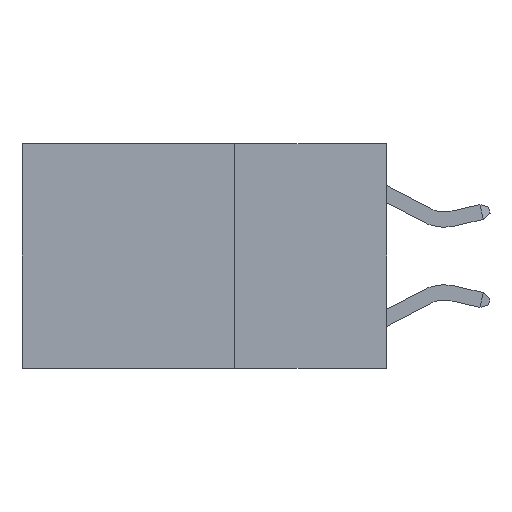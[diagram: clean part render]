
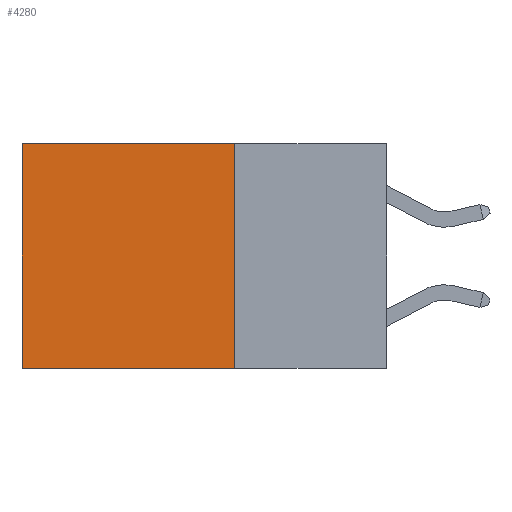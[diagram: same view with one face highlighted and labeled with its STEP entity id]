
A CAD part, left-side view. The second image highlights one B-rep face of the part: STEP entity #4280.
In plain terms, the highlighted planar face has unit normal (-1, 0, 0).
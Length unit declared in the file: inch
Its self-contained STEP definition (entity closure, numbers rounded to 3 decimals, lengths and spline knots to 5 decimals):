
#18 = ORIENTED_EDGE ( 'NONE', *, *, #11839, .F. ) ;
#91 = VERTEX_POINT ( 'NONE', #11600 ) ;
#2307 = LINE ( 'NONE', #9804, #9780 ) ;
#3784 = LINE ( 'NONE', #4873, #12627 ) ;
#3797 = CARTESIAN_POINT ( 'NONE',  ( 0.2625, 0.25, 0. ) ) ;
#4280 = ADVANCED_FACE ( 'NONE', ( #13148 ), #11788, .F. ) ;
#4529 = EDGE_CURVE ( 'NONE', #15977, #15703, #2307, .T. ) ;
#4873 = CARTESIAN_POINT ( 'NONE',  ( 0.2625, 0.25, -0.37 ) ) ;
#5460 = EDGE_CURVE ( 'NONE', #91, #15977, #6436, .T. ) ;
#5923 = ORIENTED_EDGE ( 'NONE', *, *, #5460, .T. ) ;
#6436 = LINE ( 'NONE', #3797, #9752 ) ;
#6549 = CARTESIAN_POINT ( 'NONE',  ( 0.2625, 0.6, 0. ) ) ;
#6820 = DIRECTION ( 'NONE',  ( 0., 0., -1. ) ) ;
#7505 = DIRECTION ( 'NONE',  ( 0., 0., -1. ) ) ;
#8433 = LINE ( 'NONE', #12554, #11366 ) ;
#8585 = DIRECTION ( 'NONE',  ( 0., 1., 0. ) ) ;
#8883 = DIRECTION ( 'NONE',  ( 0., 1., 0. ) ) ;
#9093 = CARTESIAN_POINT ( 'NONE',  ( 0.2625, 0.25, 0. ) ) ;
#9239 = CARTESIAN_POINT ( 'NONE',  ( 0.2625, 0.25, -0.37 ) ) ;
#9368 = EDGE_LOOP ( 'NONE', ( #12061, #18, #14628, #5923 ) ) ;
#9752 = VECTOR ( 'NONE', #8883, 39.37008 ) ;
#9780 = VECTOR ( 'NONE', #12323, 39.37008 ) ;
#9804 = CARTESIAN_POINT ( 'NONE',  ( 0.2625, 0.6, 0. ) ) ;
#11366 = VECTOR ( 'NONE', #7505, 39.37008 ) ;
#11600 = CARTESIAN_POINT ( 'NONE',  ( 0.2625, 0.25, 0. ) ) ;
#11788 = PLANE ( 'NONE',  #13014 ) ;
#11839 = EDGE_CURVE ( 'NONE', #14688, #15703, #3784, .T. ) ;
#12061 = ORIENTED_EDGE ( 'NONE', *, *, #4529, .T. ) ;
#12323 = DIRECTION ( 'NONE',  ( 0., 0., -1. ) ) ;
#12554 = CARTESIAN_POINT ( 'NONE',  ( 0.2625, 0.25, 0. ) ) ;
#12627 = VECTOR ( 'NONE', #8585, 39.37008 ) ;
#13014 = AXIS2_PLACEMENT_3D ( 'NONE', #9093, #15473, #6820 ) ;
#13148 = FACE_OUTER_BOUND ( 'NONE', #9368, .T. ) ;
#14628 = ORIENTED_EDGE ( 'NONE', *, *, #15902, .F. ) ;
#14688 = VERTEX_POINT ( 'NONE', #9239 ) ;
#15473 = DIRECTION ( 'NONE',  ( 1., 0., 0. ) ) ;
#15703 = VERTEX_POINT ( 'NONE', #16181 ) ;
#15902 = EDGE_CURVE ( 'NONE', #91, #14688, #8433, .T. ) ;
#15977 = VERTEX_POINT ( 'NONE', #6549 ) ;
#16181 = CARTESIAN_POINT ( 'NONE',  ( 0.2625, 0.6, -0.37 ) ) ;
